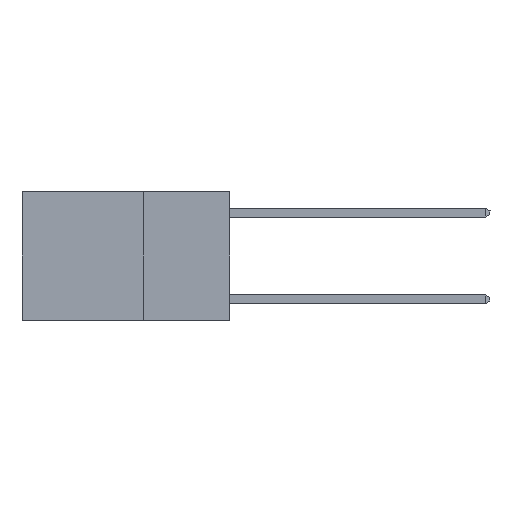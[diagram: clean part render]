
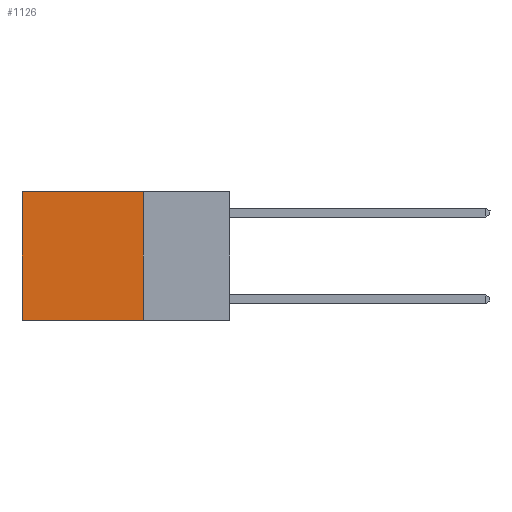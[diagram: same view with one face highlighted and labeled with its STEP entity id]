
A CAD part, left-side view. The second image highlights one B-rep face of the part: STEP entity #1126.
In plain terms, the highlighted planar face has unit normal (-1, 0, 0).
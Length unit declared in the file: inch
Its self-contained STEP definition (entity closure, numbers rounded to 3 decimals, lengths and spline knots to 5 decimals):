
#22 = CARTESIAN_POINT ( 'NONE',  ( 0.2625, 0.25, 0. ) ) ;
#594 = VECTOR ( 'NONE', #30214, 39.37008 ) ;
#1126 = ADVANCED_FACE ( 'NONE', ( #5841 ), #30729, .F. ) ;
#1649 = CARTESIAN_POINT ( 'NONE',  ( 0.2625, 0.25, 0. ) ) ;
#3332 = ORIENTED_EDGE ( 'NONE', *, *, #14257, .F. ) ;
#4068 = LINE ( 'NONE', #9105, #28182 ) ;
#4090 = DIRECTION ( 'NONE',  ( 0., 0., -1. ) ) ;
#4802 = CARTESIAN_POINT ( 'NONE',  ( 0.2625, 0.6, -0.37 ) ) ;
#5841 = FACE_OUTER_BOUND ( 'NONE', #6078, .T. ) ;
#6078 = EDGE_LOOP ( 'NONE', ( #20714, #25833, #3332, #29924 ) ) ;
#7771 = EDGE_CURVE ( 'NONE', #20701, #11376, #12847, .T. ) ;
#8667 = LINE ( 'NONE', #1649, #27863 ) ;
#8733 = VERTEX_POINT ( 'NONE', #22 ) ;
#8974 = VERTEX_POINT ( 'NONE', #29877 ) ;
#9105 = CARTESIAN_POINT ( 'NONE',  ( 0.2625, 0.6, 0. ) ) ;
#11376 = VERTEX_POINT ( 'NONE', #4802 ) ;
#11534 = DIRECTION ( 'NONE',  ( 0., 0., -1. ) ) ;
#12847 = LINE ( 'NONE', #13405, #594 ) ;
#13405 = CARTESIAN_POINT ( 'NONE',  ( 0.2625, 0.25, -0.37 ) ) ;
#14006 = DIRECTION ( 'NONE',  ( 1., 0., 0. ) ) ;
#14257 = EDGE_CURVE ( 'NONE', #8733, #20701, #8667, .T. ) ;
#16320 = LINE ( 'NONE', #18182, #26845 ) ;
#17919 = EDGE_CURVE ( 'NONE', #8974, #11376, #4068, .T. ) ;
#18182 = CARTESIAN_POINT ( 'NONE',  ( 0.2625, 0.25, 0. ) ) ;
#20701 = VERTEX_POINT ( 'NONE', #26602 ) ;
#20714 = ORIENTED_EDGE ( 'NONE', *, *, #17919, .T. ) ;
#23543 = CARTESIAN_POINT ( 'NONE',  ( 0.2625, 0.25, 0. ) ) ;
#25423 = DIRECTION ( 'NONE',  ( 0., 1., 0. ) ) ;
#25833 = ORIENTED_EDGE ( 'NONE', *, *, #7771, .F. ) ;
#25838 = AXIS2_PLACEMENT_3D ( 'NONE', #23543, #14006, #30838 ) ;
#26602 = CARTESIAN_POINT ( 'NONE',  ( 0.2625, 0.25, -0.37 ) ) ;
#26845 = VECTOR ( 'NONE', #25423, 39.37008 ) ;
#27355 = EDGE_CURVE ( 'NONE', #8733, #8974, #16320, .T. ) ;
#27863 = VECTOR ( 'NONE', #4090, 39.37008 ) ;
#28182 = VECTOR ( 'NONE', #11534, 39.37008 ) ;
#29877 = CARTESIAN_POINT ( 'NONE',  ( 0.2625, 0.6, 0. ) ) ;
#29924 = ORIENTED_EDGE ( 'NONE', *, *, #27355, .T. ) ;
#30214 = DIRECTION ( 'NONE',  ( 0., 1., 0. ) ) ;
#30729 = PLANE ( 'NONE',  #25838 ) ;
#30838 = DIRECTION ( 'NONE',  ( 0., 0., -1. ) ) ;
